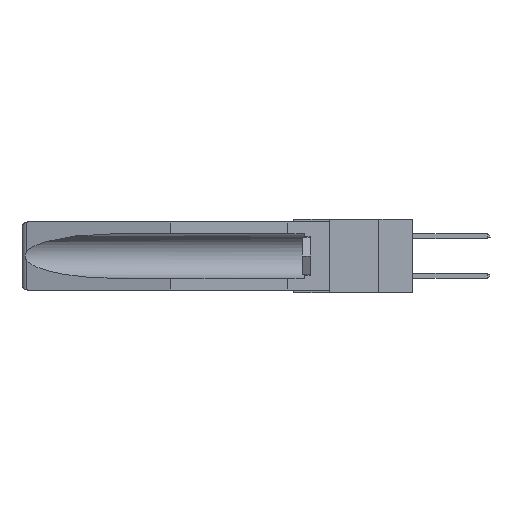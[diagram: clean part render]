
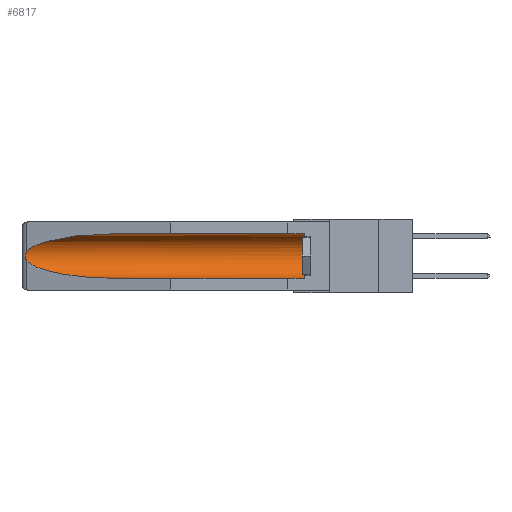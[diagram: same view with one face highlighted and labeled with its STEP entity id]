
A CAD part, left-side view. The second image highlights one B-rep face of the part: STEP entity #6817.
In plain terms, the highlighted cylindrical face has radius 2.857 mm (diameter 5.715 mm), a partial arc.
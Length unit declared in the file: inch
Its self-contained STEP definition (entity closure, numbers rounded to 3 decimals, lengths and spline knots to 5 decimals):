
#1064 = ORIENTED_EDGE ( 'NONE', *, *, #22667, .T. ) ;
#1629 = CARTESIAN_POINT ( 'NONE',  ( 0.26597, 1.5296, -0.19026 ) ) ;
#1649 = DIRECTION ( 'NONE',  ( 0., -1., 0. ) ) ;
#2238 = B_SPLINE_CURVE_WITH_KNOTS ( 'NONE', 3,
 ( #11174, #28872, #29092, #19090, #6540, #28766, #18762, #8718, #1629, #6869 ),
 .UNSPECIFIED., .F., .F.,
 ( 4, 2, 2, 2, 4 ),
 ( 0., 0.00029, 0.00058, 0.00087, 0.00117 ),
 .UNSPECIFIED. ) ;
#2476 = AXIS2_PLACEMENT_3D ( 'NONE', #14625, #1649, #6885 ) ;
#3047 = VERTEX_POINT ( 'NONE', #15320 ) ;
#4567 = CARTESIAN_POINT ( 'NONE',  ( 0.155, 1.07973, -0.284 ) ) ;
#4625 = CYLINDRICAL_SURFACE ( 'NONE', #18477, 0.1125 ) ;
#5884 = CIRCLE ( 'NONE', #2476, 0.1125 ) ;
#6540 = CARTESIAN_POINT ( 'NONE',  ( 0.2675, 1.53308, -0.16763 ) ) ;
#6713 = CARTESIAN_POINT ( 'NONE',  ( 0.25451, 1.48313, -0.09465 ) ) ;
#6817 = ADVANCED_FACE ( 'NONE', ( #27917 ), #4625, .F. ) ;
#6869 = CARTESIAN_POINT ( 'NONE',  ( 0.26537, 1.52718, -0.19328 ) ) ;
#6885 = DIRECTION ( 'NONE',  ( 0., 0., 1. ) ) ;
#7443 = CARTESIAN_POINT ( 'NONE',  ( 0.25451, 1.48313, -0.24835 ) ) ;
#7516 =( BOUNDED_CURVE ( )  B_SPLINE_CURVE ( 3, ( #21668, #14221, #6713, #26867 ),
 .UNSPECIFIED., .F., .F. ) 
 B_SPLINE_CURVE_WITH_KNOTS ( ( 4, 4 ),
 ( 4.71239, 6.08839 ),
 .UNSPECIFIED. ) 
 CURVE ( )  GEOMETRIC_REPRESENTATION_ITEM ( )  RATIONAL_B_SPLINE_CURVE ( ( 1., 0.848, 0.848, 1. ) ) 
 REPRESENTATION_ITEM ( '' )  );
#8718 = CARTESIAN_POINT ( 'NONE',  ( 0.26655, 1.53094, -0.18657 ) ) ;
#8910 = VERTEX_POINT ( 'NONE', #10652 ) ;
#9222 = DIRECTION ( 'NONE',  ( 0., 1., 0. ) ) ;
#9507 = VECTOR ( 'NONE', #15411, 39.37008 ) ;
#10652 = CARTESIAN_POINT ( 'NONE',  ( 0.155, 0.126, -0.059 ) ) ;
#10961 = VERTEX_POINT ( 'NONE', #18967 ) ;
#11109 = LINE ( 'NONE', #15523, #9507 ) ;
#11174 = CARTESIAN_POINT ( 'NONE',  ( 0.26537, 1.52718, -0.14972 ) ) ;
#12232 = ORIENTED_EDGE ( 'NONE', *, *, #25523, .T. ) ;
#13328 = CARTESIAN_POINT ( 'NONE',  ( 0.26537, 1.52718, -0.14972 ) ) ;
#13518 = VERTEX_POINT ( 'NONE', #13328 ) ;
#14221 = CARTESIAN_POINT ( 'NONE',  ( 0.21114, 1.30732, -0.059 ) ) ;
#14326 = CARTESIAN_POINT ( 'NONE',  ( 0.155, -0.30754, -0.1715 ) ) ;
#14625 = CARTESIAN_POINT ( 'NONE',  ( 0.155, 0.126, -0.1715 ) ) ;
#14675 = LINE ( 'NONE', #19225, #26838 ) ;
#15320 = CARTESIAN_POINT ( 'NONE',  ( 0.26537, 1.52718, -0.19328 ) ) ;
#15411 = DIRECTION ( 'NONE',  ( 0., 1., 0. ) ) ;
#15523 = CARTESIAN_POINT ( 'NONE',  ( 0.155, -0.30754, -0.284 ) ) ;
#16230 = CARTESIAN_POINT ( 'NONE',  ( 0.155, 0.126, -0.284 ) ) ;
#16237 = ORIENTED_EDGE ( 'NONE', *, *, #22977, .T. ) ;
#16602 = VERTEX_POINT ( 'NONE', #16230 ) ;
#18477 = AXIS2_PLACEMENT_3D ( 'NONE', #14326, #9222, #24408 ) ;
#18762 = CARTESIAN_POINT ( 'NONE',  ( 0.2673, 1.53269, -0.17917 ) ) ;
#18967 = CARTESIAN_POINT ( 'NONE',  ( 0.155, 1.07973, -0.059 ) ) ;
#19090 = CARTESIAN_POINT ( 'NONE',  ( 0.2673, 1.5327, -0.16383 ) ) ;
#19225 = CARTESIAN_POINT ( 'NONE',  ( 0.155, -0.30754, -0.059 ) ) ;
#21179 = ORIENTED_EDGE ( 'NONE', *, *, #25163, .T. ) ;
#21567 = CARTESIAN_POINT ( 'NONE',  ( 0.155, 1.07973, -0.284 ) ) ;
#21668 = CARTESIAN_POINT ( 'NONE',  ( 0.155, 1.07973, -0.059 ) ) ;
#21957 = EDGE_CURVE ( 'NONE', #16602, #23937, #11109, .T. ) ;
#22270 =( BOUNDED_CURVE ( )  B_SPLINE_CURVE ( 3, ( #22340, #7443, #32207, #4567 ),
 .UNSPECIFIED., .F., .F. ) 
 B_SPLINE_CURVE_WITH_KNOTS ( ( 4, 4 ),
 ( 0.1948, 1.5708 ),
 .UNSPECIFIED. ) 
 CURVE ( )  GEOMETRIC_REPRESENTATION_ITEM ( )  RATIONAL_B_SPLINE_CURVE ( ( 1., 0.848, 0.848, 1. ) ) 
 REPRESENTATION_ITEM ( '' )  );
#22340 = CARTESIAN_POINT ( 'NONE',  ( 0.26537, 1.52718, -0.19328 ) ) ;
#22434 = EDGE_CURVE ( 'NONE', #8910, #10961, #14675, .T. ) ;
#22667 = EDGE_CURVE ( 'NONE', #10961, #13518, #7516, .T. ) ;
#22977 = EDGE_CURVE ( 'NONE', #16602, #8910, #5884, .T. ) ;
#23878 = ORIENTED_EDGE ( 'NONE', *, *, #21957, .F. ) ;
#23937 = VERTEX_POINT ( 'NONE', #21567 ) ;
#24408 = DIRECTION ( 'NONE',  ( 0., 0., 1. ) ) ;
#25163 = EDGE_CURVE ( 'NONE', #3047, #23937, #22270, .T. ) ;
#25523 = EDGE_CURVE ( 'NONE', #13518, #3047, #2238, .T. ) ;
#26838 = VECTOR ( 'NONE', #29317, 39.37008 ) ;
#26867 = CARTESIAN_POINT ( 'NONE',  ( 0.26537, 1.52718, -0.14972 ) ) ;
#27917 = FACE_OUTER_BOUND ( 'NONE', #29167, .T. ) ;
#28216 = ORIENTED_EDGE ( 'NONE', *, *, #22434, .T. ) ;
#28766 = CARTESIAN_POINT ( 'NONE',  ( 0.2675, 1.53308, -0.17534 ) ) ;
#28872 = CARTESIAN_POINT ( 'NONE',  ( 0.26597, 1.52961, -0.15275 ) ) ;
#29092 = CARTESIAN_POINT ( 'NONE',  ( 0.26654, 1.53092, -0.15636 ) ) ;
#29167 = EDGE_LOOP ( 'NONE', ( #1064, #12232, #21179, #23878, #16237, #28216 ) ) ;
#29317 = DIRECTION ( 'NONE',  ( 0., 1., 0. ) ) ;
#32207 = CARTESIAN_POINT ( 'NONE',  ( 0.21114, 1.30732, -0.284 ) ) ;
